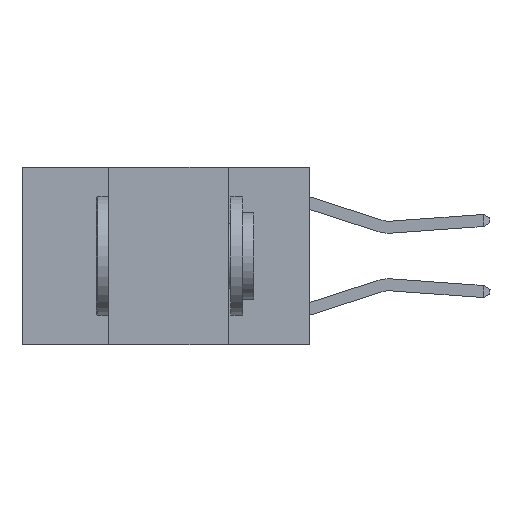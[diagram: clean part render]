
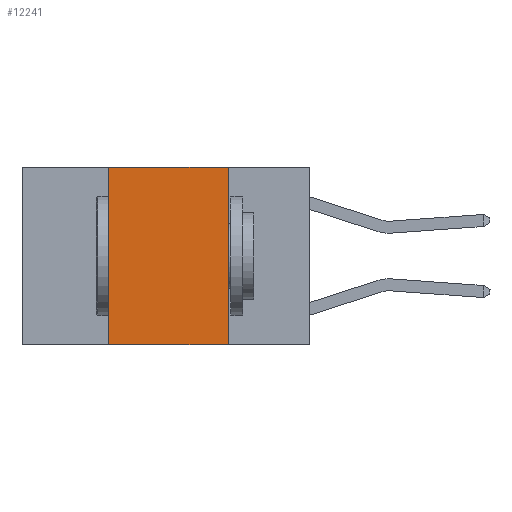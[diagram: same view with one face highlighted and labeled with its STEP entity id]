
A CAD part, left-side view. The second image highlights one B-rep face of the part: STEP entity #12241.
In plain terms, the highlighted planar face has unit normal (-1, 0, 0).
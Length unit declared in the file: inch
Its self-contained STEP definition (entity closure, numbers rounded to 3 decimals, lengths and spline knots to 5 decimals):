
#396 = ORIENTED_EDGE ( 'NONE', *, *, #2537, .F. ) ;
#1731 = VECTOR ( 'NONE', #15466, 39.37008 ) ;
#1862 = VERTEX_POINT ( 'NONE', #7353 ) ;
#2260 = EDGE_CURVE ( 'NONE', #1862, #13143, #8623, .T. ) ;
#2388 = CARTESIAN_POINT ( 'NONE',  ( 0., 0.6, 0. ) ) ;
#2537 = EDGE_CURVE ( 'NONE', #13143, #2833, #15429, .T. ) ;
#2783 = EDGE_CURVE ( 'NONE', #12471, #1862, #5086, .T. ) ;
#2833 = VERTEX_POINT ( 'NONE', #7904 ) ;
#3612 = DIRECTION ( 'NONE',  ( 1., 0., 0. ) ) ;
#3625 = VECTOR ( 'NONE', #6132, 39.37008 ) ;
#3705 = CARTESIAN_POINT ( 'NONE',  ( 0., 0.6, -0.37 ) ) ;
#4919 = CARTESIAN_POINT ( 'NONE',  ( 0., 0.17, 0. ) ) ;
#5086 = LINE ( 'NONE', #7748, #7949 ) ;
#6132 = DIRECTION ( 'NONE',  ( 0., -1., 0. ) ) ;
#6558 = DIRECTION ( 'NONE',  ( 0., 0., 1. ) ) ;
#7165 = ORIENTED_EDGE ( 'NONE', *, *, #13450, .T. ) ;
#7353 = CARTESIAN_POINT ( 'NONE',  ( 0., 0.42, 0. ) ) ;
#7748 = CARTESIAN_POINT ( 'NONE',  ( 0., 0.42, 0. ) ) ;
#7904 = CARTESIAN_POINT ( 'NONE',  ( 0., 0.17, -0.37 ) ) ;
#7949 = VECTOR ( 'NONE', #6558, 39.37008 ) ;
#8233 = FACE_OUTER_BOUND ( 'NONE', #11860, .T. ) ;
#8623 = LINE ( 'NONE', #13018, #1731 ) ;
#8866 = AXIS2_PLACEMENT_3D ( 'NONE', #2388, #3612, #12160 ) ;
#9700 = PLANE ( 'NONE',  #8866 ) ;
#10112 = LINE ( 'NONE', #3705, #3625 ) ;
#10964 = ORIENTED_EDGE ( 'NONE', *, *, #2260, .F. ) ;
#11653 = CARTESIAN_POINT ( 'NONE',  ( 0., 0.17, 0. ) ) ;
#11860 = EDGE_LOOP ( 'NONE', ( #396, #10964, #12986, #7165 ) ) ;
#12160 = DIRECTION ( 'NONE',  ( 0., 0., -1. ) ) ;
#12197 = DIRECTION ( 'NONE',  ( 0., 0., -1. ) ) ;
#12241 = ADVANCED_FACE ( 'NONE', ( #8233 ), #9700, .F. ) ;
#12471 = VERTEX_POINT ( 'NONE', #13891 ) ;
#12986 = ORIENTED_EDGE ( 'NONE', *, *, #2783, .F. ) ;
#13018 = CARTESIAN_POINT ( 'NONE',  ( 0., 0.6, 0. ) ) ;
#13143 = VERTEX_POINT ( 'NONE', #11653 ) ;
#13450 = EDGE_CURVE ( 'NONE', #12471, #2833, #10112, .T. ) ;
#13891 = CARTESIAN_POINT ( 'NONE',  ( 0., 0.42, -0.37 ) ) ;
#14663 = VECTOR ( 'NONE', #12197, 39.37008 ) ;
#15429 = LINE ( 'NONE', #4919, #14663 ) ;
#15466 = DIRECTION ( 'NONE',  ( 0., -1., 0. ) ) ;
